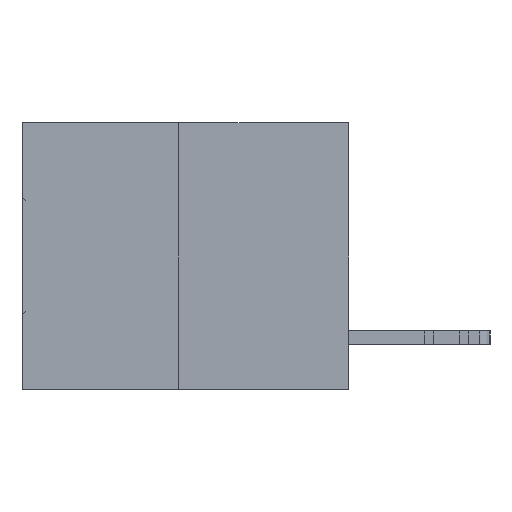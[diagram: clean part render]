
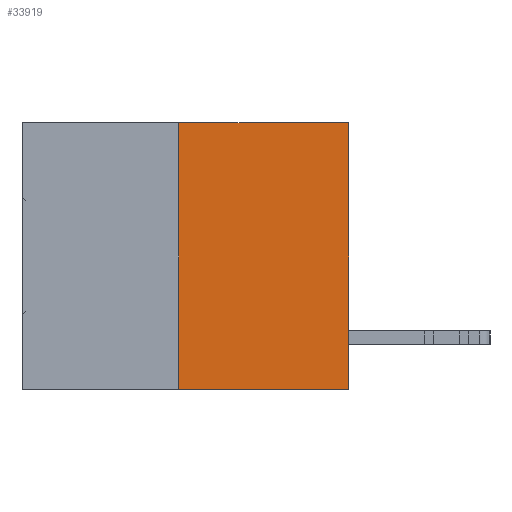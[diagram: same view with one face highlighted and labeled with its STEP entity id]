
A CAD part, left-side view. The second image highlights one B-rep face of the part: STEP entity #33919.
In plain terms, the highlighted planar face has unit normal (-1, 0, 0).
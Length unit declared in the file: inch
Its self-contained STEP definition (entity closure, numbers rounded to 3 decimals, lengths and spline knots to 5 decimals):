
#453 = LINE ( 'NONE', #34272, #30022 ) ;
#948 = VERTEX_POINT ( 'NONE', #30507 ) ;
#1450 = DIRECTION ( 'NONE',  ( 0., 0., 1. ) ) ;
#3417 = DIRECTION ( 'NONE',  ( 0., -1., 0. ) ) ;
#3548 = CARTESIAN_POINT ( 'NONE',  ( 0., 0.312, -0.49 ) ) ;
#4296 = ORIENTED_EDGE ( 'NONE', *, *, #29007, .T. ) ;
#5001 = LINE ( 'NONE', #3548, #15655 ) ;
#6577 = PLANE ( 'NONE',  #25390 ) ;
#8578 = DIRECTION ( 'NONE',  ( 0., -1., 0. ) ) ;
#9308 = DIRECTION ( 'NONE',  ( 1., 0., 0. ) ) ;
#9500 = CARTESIAN_POINT ( 'NONE',  ( 0., 0., 0. ) ) ;
#11326 = FACE_OUTER_BOUND ( 'NONE', #34137, .T. ) ;
#12081 = DIRECTION ( 'NONE',  ( 0., 0., -1. ) ) ;
#12205 = CARTESIAN_POINT ( 'NONE',  ( 0., 0.6, 0. ) ) ;
#12334 = VERTEX_POINT ( 'NONE', #17400 ) ;
#13014 = LINE ( 'NONE', #14304, #31891 ) ;
#13018 = EDGE_CURVE ( 'NONE', #948, #12334, #5001, .T. ) ;
#13110 = ORIENTED_EDGE ( 'NONE', *, *, #34331, .F. ) ;
#13857 = CARTESIAN_POINT ( 'NONE',  ( 0., 0.6, -0.49 ) ) ;
#14304 = CARTESIAN_POINT ( 'NONE',  ( 0., 0.6, 0. ) ) ;
#15655 = VECTOR ( 'NONE', #26539, 39.37008 ) ;
#17400 = CARTESIAN_POINT ( 'NONE',  ( 0., 0.312, 0. ) ) ;
#17510 = EDGE_CURVE ( 'NONE', #20042, #33378, #453, .T. ) ;
#18850 = LINE ( 'NONE', #13857, #24904 ) ;
#20042 = VERTEX_POINT ( 'NONE', #21766 ) ;
#21766 = CARTESIAN_POINT ( 'NONE',  ( 0., 0., -0.49 ) ) ;
#24904 = VECTOR ( 'NONE', #8578, 39.37008 ) ;
#25390 = AXIS2_PLACEMENT_3D ( 'NONE', #12205, #9308, #12081 ) ;
#26539 = DIRECTION ( 'NONE',  ( 0., 0., 1. ) ) ;
#28850 = ORIENTED_EDGE ( 'NONE', *, *, #13018, .F. ) ;
#29007 = EDGE_CURVE ( 'NONE', #948, #20042, #18850, .T. ) ;
#30022 = VECTOR ( 'NONE', #1450, 39.37008 ) ;
#30507 = CARTESIAN_POINT ( 'NONE',  ( 0., 0.312, -0.49 ) ) ;
#31891 = VECTOR ( 'NONE', #3417, 39.37008 ) ;
#32131 = ORIENTED_EDGE ( 'NONE', *, *, #17510, .T. ) ;
#33378 = VERTEX_POINT ( 'NONE', #9500 ) ;
#33919 = ADVANCED_FACE ( 'NONE', ( #11326 ), #6577, .F. ) ;
#34137 = EDGE_LOOP ( 'NONE', ( #28850, #4296, #32131, #13110 ) ) ;
#34272 = CARTESIAN_POINT ( 'NONE',  ( 0., 0., 0. ) ) ;
#34331 = EDGE_CURVE ( 'NONE', #12334, #33378, #13014, .T. ) ;
